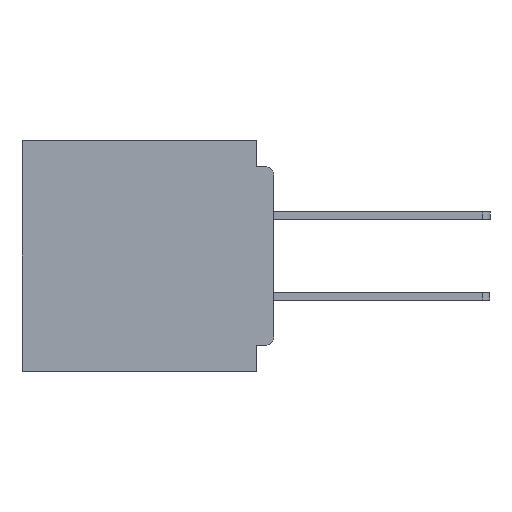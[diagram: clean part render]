
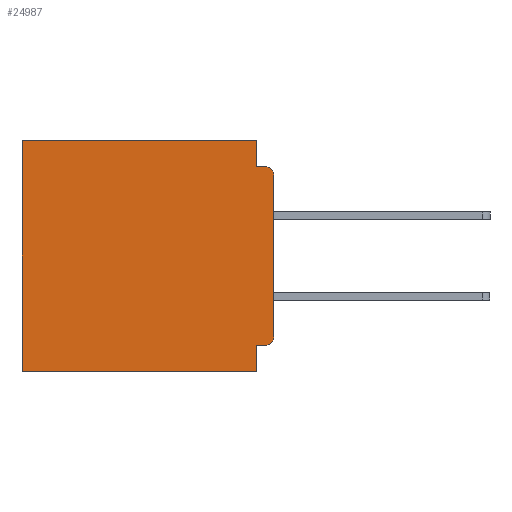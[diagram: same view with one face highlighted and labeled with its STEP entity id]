
A CAD part, left-side view. The second image highlights one B-rep face of the part: STEP entity #24987.
In plain terms, the highlighted planar face has unit normal (-1, 0, 0).
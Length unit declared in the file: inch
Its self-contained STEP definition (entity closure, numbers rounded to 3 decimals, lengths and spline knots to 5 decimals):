
#1303 = VERTEX_POINT ( 'NONE', #20419 ) ;
#2345 = DIRECTION ( 'NONE',  ( -1., 0., 0. ) ) ;
#2778 = CARTESIAN_POINT ( 'NONE',  ( 0.3, 0., -0.4 ) ) ;
#3547 = EDGE_CURVE ( 'NONE', #41871, #35624, #30817, .T. ) ;
#4466 = DIRECTION ( 'NONE',  ( 0., 0., -1. ) ) ;
#7164 = EDGE_CURVE ( 'NONE', #47706, #20066, #39977, .T. ) ;
#7957 = CARTESIAN_POINT ( 'NONE',  ( 0.3, 0., -0.34 ) ) ;
#8610 = AXIS2_PLACEMENT_3D ( 'NONE', #11710, #42097, #16045 ) ;
#10065 = DIRECTION ( 'NONE',  ( 0., 1., 0. ) ) ;
#10539 = VECTOR ( 'NONE', #4466, 39.37008 ) ;
#11197 = CARTESIAN_POINT ( 'NONE',  ( 0.3, 0.031, 0. ) ) ;
#11710 = CARTESIAN_POINT ( 'NONE',  ( 0.3, 0.015, -0.34 ) ) ;
#12397 = CARTESIAN_POINT ( 'NONE',  ( 0.3, 0.015, -0.355 ) ) ;
#13549 = VERTEX_POINT ( 'NONE', #41717 ) ;
#14543 = CIRCLE ( 'NONE', #14622, 0.015 ) ;
#14622 = AXIS2_PLACEMENT_3D ( 'NONE', #28434, #2345, #32859 ) ;
#14789 = VECTOR ( 'NONE', #17917, 39.37008 ) ;
#14874 = EDGE_LOOP ( 'NONE', ( #17792, #18388, #18551, #18815, #19572, #19796, #20598, #21537, #21897, #22264 ) ) ;
#15416 = VECTOR ( 'NONE', #10065, 39.37008 ) ;
#16045 = DIRECTION ( 'NONE',  ( 0., 0., -1. ) ) ;
#16147 = LINE ( 'NONE', #26507, #14789 ) ;
#17021 = CARTESIAN_POINT ( 'NONE',  ( 0.3, 0., -0.4 ) ) ;
#17792 = ORIENTED_EDGE ( 'NONE', *, *, #19533, .F. ) ;
#17903 = CARTESIAN_POINT ( 'NONE',  ( 0.3, 0.031, -0.045 ) ) ;
#17917 = DIRECTION ( 'NONE',  ( 0., 0., -1. ) ) ;
#18297 = CARTESIAN_POINT ( 'NONE',  ( 0.3, 0.437, 0. ) ) ;
#18388 = ORIENTED_EDGE ( 'NONE', *, *, #19857, .T. ) ;
#18551 = ORIENTED_EDGE ( 'NONE', *, *, #29418, .F. ) ;
#18815 = ORIENTED_EDGE ( 'NONE', *, *, #40184, .F. ) ;
#19533 = EDGE_CURVE ( 'NONE', #1303, #52851, #20700, .T. ) ;
#19572 = ORIENTED_EDGE ( 'NONE', *, *, #44828, .T. ) ;
#19796 = ORIENTED_EDGE ( 'NONE', *, *, #3547, .T. ) ;
#19857 = EDGE_CURVE ( 'NONE', #1303, #13549, #14543, .T. ) ;
#20066 = VERTEX_POINT ( 'NONE', #37258 ) ;
#20281 = AXIS2_PLACEMENT_3D ( 'NONE', #17021, #47309, #21409 ) ;
#20419 = CARTESIAN_POINT ( 'NONE',  ( 0.3, 0., -0.06 ) ) ;
#20598 = ORIENTED_EDGE ( 'NONE', *, *, #21986, .F. ) ;
#20700 = LINE ( 'NONE', #34970, #10539 ) ;
#21295 = VECTOR ( 'NONE', #37650, 39.37008 ) ;
#21409 = DIRECTION ( 'NONE',  ( 0., 0., -1. ) ) ;
#21537 = ORIENTED_EDGE ( 'NONE', *, *, #55393, .F. ) ;
#21897 = ORIENTED_EDGE ( 'NONE', *, *, #7164, .F. ) ;
#21986 = EDGE_CURVE ( 'NONE', #52603, #35624, #43017, .T. ) ;
#22264 = ORIENTED_EDGE ( 'NONE', *, *, #47034, .T. ) ;
#23791 = CARTESIAN_POINT ( 'NONE',  ( 0.3, 0.437, -0.4 ) ) ;
#23856 = CARTESIAN_POINT ( 'NONE',  ( 0.3, 0.031, -0.4 ) ) ;
#24987 = ADVANCED_FACE ( 'NONE', ( #34733 ), #34443, .F. ) ;
#26507 = CARTESIAN_POINT ( 'NONE',  ( 0.3, 0.031, 0. ) ) ;
#28434 = CARTESIAN_POINT ( 'NONE',  ( 0.3, 0.015, -0.06 ) ) ;
#29418 = EDGE_CURVE ( 'NONE', #37321, #13549, #47716, .T. ) ;
#30709 = LINE ( 'NONE', #32594, #52128 ) ;
#30817 = LINE ( 'NONE', #42105, #53525 ) ;
#32315 = VECTOR ( 'NONE', #48772, 39.37008 ) ;
#32594 = CARTESIAN_POINT ( 'NONE',  ( 0.3, 0., 0. ) ) ;
#32772 = CARTESIAN_POINT ( 'NONE',  ( 0.3, 0.031, -0.4 ) ) ;
#32859 = DIRECTION ( 'NONE',  ( 0., 0., -1. ) ) ;
#34443 = PLANE ( 'NONE',  #20281 ) ;
#34677 = VECTOR ( 'NONE', #45597, 39.37008 ) ;
#34733 = FACE_OUTER_BOUND ( 'NONE', #14874, .T. ) ;
#34970 = CARTESIAN_POINT ( 'NONE',  ( 0.3, 0., -0.4 ) ) ;
#35624 = VERTEX_POINT ( 'NONE', #23791 ) ;
#36156 = CARTESIAN_POINT ( 'NONE',  ( 0.3, 0., -0.355 ) ) ;
#37258 = CARTESIAN_POINT ( 'NONE',  ( 0.3, 0.031, -0.355 ) ) ;
#37321 = VERTEX_POINT ( 'NONE', #17903 ) ;
#37383 = LINE ( 'NONE', #23856, #34677 ) ;
#37650 = DIRECTION ( 'NONE',  ( 0., 1., 0. ) ) ;
#39977 = LINE ( 'NONE', #36156, #15416 ) ;
#40184 = EDGE_CURVE ( 'NONE', #52665, #37321, #16147, .T. ) ;
#40768 = DIRECTION ( 'NONE',  ( 0., 0., -1. ) ) ;
#41717 = CARTESIAN_POINT ( 'NONE',  ( 0.3, 0.015, -0.045 ) ) ;
#41871 = VERTEX_POINT ( 'NONE', #18297 ) ;
#42097 = DIRECTION ( 'NONE',  ( -1., 0., 0. ) ) ;
#42105 = CARTESIAN_POINT ( 'NONE',  ( 0.3, 0.437, -0.4 ) ) ;
#43017 = LINE ( 'NONE', #2778, #21295 ) ;
#44488 = CARTESIAN_POINT ( 'NONE',  ( 0.3, 0., -0.045 ) ) ;
#44828 = EDGE_CURVE ( 'NONE', #52665, #41871, #30709, .T. ) ;
#45597 = DIRECTION ( 'NONE',  ( 0., 0., -1. ) ) ;
#47034 = EDGE_CURVE ( 'NONE', #47706, #52851, #47436, .T. ) ;
#47309 = DIRECTION ( 'NONE',  ( 1., 0., 0. ) ) ;
#47436 = CIRCLE ( 'NONE', #8610, 0.015 ) ;
#47706 = VERTEX_POINT ( 'NONE', #12397 ) ;
#47716 = LINE ( 'NONE', #44488, #32315 ) ;
#48772 = DIRECTION ( 'NONE',  ( 0., -1., 0. ) ) ;
#49786 = DIRECTION ( 'NONE',  ( 0., 1., 0. ) ) ;
#52128 = VECTOR ( 'NONE', #49786, 39.37008 ) ;
#52603 = VERTEX_POINT ( 'NONE', #32772 ) ;
#52665 = VERTEX_POINT ( 'NONE', #11197 ) ;
#52851 = VERTEX_POINT ( 'NONE', #7957 ) ;
#53525 = VECTOR ( 'NONE', #40768, 39.37008 ) ;
#55393 = EDGE_CURVE ( 'NONE', #20066, #52603, #37383, .T. ) ;
